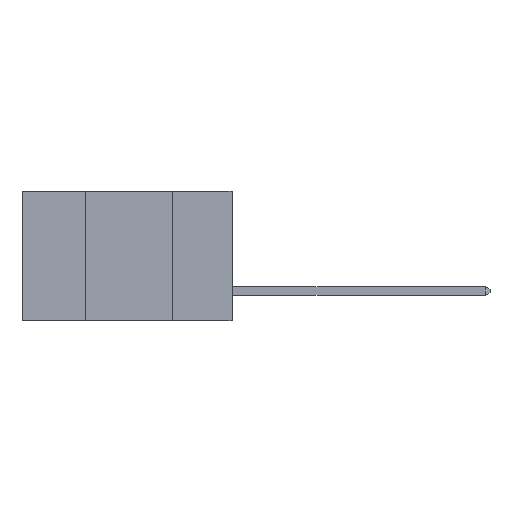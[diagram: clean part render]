
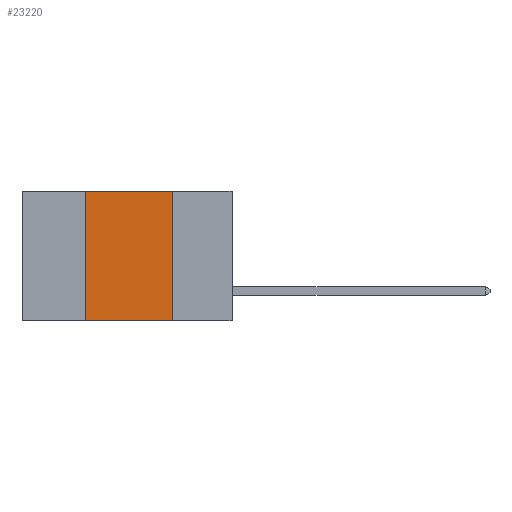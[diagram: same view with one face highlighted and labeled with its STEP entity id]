
A CAD part, left-side view. The second image highlights one B-rep face of the part: STEP entity #23220.
In plain terms, the highlighted planar face has unit normal (-1, 0, 0).
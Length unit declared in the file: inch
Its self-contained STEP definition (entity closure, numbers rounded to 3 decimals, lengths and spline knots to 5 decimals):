
#38 = VERTEX_POINT ( 'NONE', #3793 ) ;
#212 = EDGE_LOOP ( 'NONE', ( #3232, #3835, #14282, #599 ) ) ;
#515 = VECTOR ( 'NONE', #18096, 39.37008 ) ;
#599 = ORIENTED_EDGE ( 'NONE', *, *, #17686, .T. ) ;
#2433 = CARTESIAN_POINT ( 'NONE',  ( 0., 0.42, -0.37 ) ) ;
#2745 = DIRECTION ( 'NONE',  ( 0., 0., 1. ) ) ;
#3232 = ORIENTED_EDGE ( 'NONE', *, *, #19009, .F. ) ;
#3793 = CARTESIAN_POINT ( 'NONE',  ( 0., 0.17, 0. ) ) ;
#3835 = ORIENTED_EDGE ( 'NONE', *, *, #4845, .F. ) ;
#4845 = EDGE_CURVE ( 'NONE', #13299, #38, #14870, .T. ) ;
#5207 = CARTESIAN_POINT ( 'NONE',  ( 0., 0.6, 0. ) ) ;
#5227 = CARTESIAN_POINT ( 'NONE',  ( 0., 0.17, 0. ) ) ;
#5543 = LINE ( 'NONE', #5227, #515 ) ;
#5714 = VERTEX_POINT ( 'NONE', #15537 ) ;
#7067 = EDGE_CURVE ( 'NONE', #20132, #13299, #10165, .T. ) ;
#7083 = DIRECTION ( 'NONE',  ( 1., 0., 0. ) ) ;
#8301 = CARTESIAN_POINT ( 'NONE',  ( 0., 0.42, 0. ) ) ;
#8602 = DIRECTION ( 'NONE',  ( 0., -1., 0. ) ) ;
#9553 = DIRECTION ( 'NONE',  ( 0., -1., 0. ) ) ;
#9634 = CARTESIAN_POINT ( 'NONE',  ( 0., 0.6, 0. ) ) ;
#9965 = VECTOR ( 'NONE', #9553, 39.37008 ) ;
#10165 = LINE ( 'NONE', #8301, #23434 ) ;
#12535 = PLANE ( 'NONE',  #17823 ) ;
#13299 = VERTEX_POINT ( 'NONE', #14227 ) ;
#14227 = CARTESIAN_POINT ( 'NONE',  ( 0., 0.42, 0. ) ) ;
#14282 = ORIENTED_EDGE ( 'NONE', *, *, #7067, .F. ) ;
#14870 = LINE ( 'NONE', #9634, #9965 ) ;
#15537 = CARTESIAN_POINT ( 'NONE',  ( 0., 0.17, -0.37 ) ) ;
#17686 = EDGE_CURVE ( 'NONE', #20132, #5714, #21865, .T. ) ;
#17765 = CARTESIAN_POINT ( 'NONE',  ( 0., 0.6, -0.37 ) ) ;
#17823 = AXIS2_PLACEMENT_3D ( 'NONE', #5207, #7083, #19843 ) ;
#18096 = DIRECTION ( 'NONE',  ( 0., 0., -1. ) ) ;
#19009 = EDGE_CURVE ( 'NONE', #38, #5714, #5543, .T. ) ;
#19843 = DIRECTION ( 'NONE',  ( 0., 0., -1. ) ) ;
#20132 = VERTEX_POINT ( 'NONE', #2433 ) ;
#21310 = VECTOR ( 'NONE', #8602, 39.37008 ) ;
#21865 = LINE ( 'NONE', #17765, #21310 ) ;
#22795 = FACE_OUTER_BOUND ( 'NONE', #212, .T. ) ;
#23220 = ADVANCED_FACE ( 'NONE', ( #22795 ), #12535, .F. ) ;
#23434 = VECTOR ( 'NONE', #2745, 39.37008 ) ;
